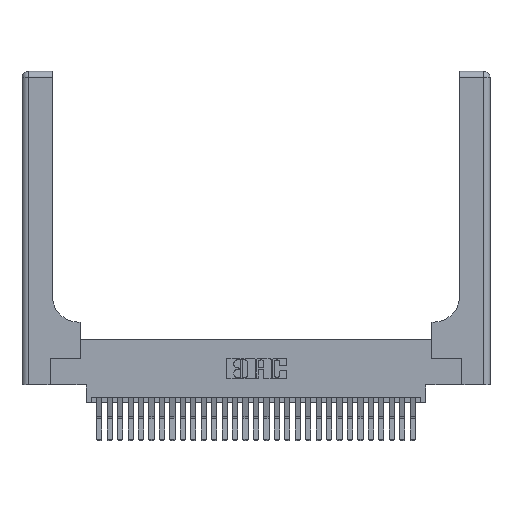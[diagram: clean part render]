
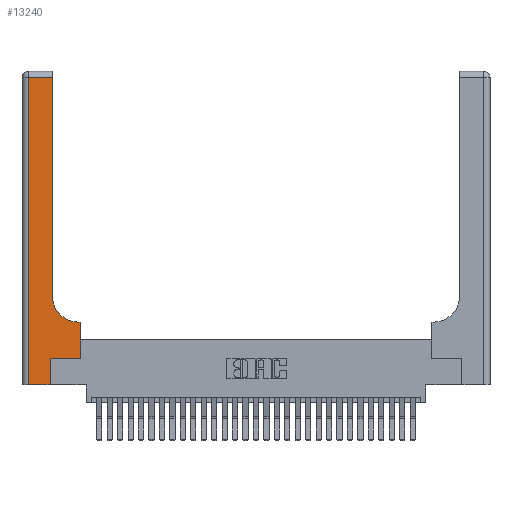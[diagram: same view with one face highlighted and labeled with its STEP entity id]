
A CAD part, top view. The second image highlights one B-rep face of the part: STEP entity #13240.
In plain terms, the highlighted planar face has unit normal (0, 0, 1).
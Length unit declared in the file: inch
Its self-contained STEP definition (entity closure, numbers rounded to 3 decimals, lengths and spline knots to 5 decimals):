
#451 = DIRECTION ( 'NONE',  ( 0., 1., 0. ) ) ;
#740 = VERTEX_POINT ( 'NONE', #11232 ) ;
#1038 = VERTEX_POINT ( 'NONE', #19438 ) ;
#1627 = CARTESIAN_POINT ( 'NONE',  ( 0.5585, 0.25, 0.37 ) ) ;
#1645 = CARTESIAN_POINT ( 'NONE',  ( 0.2915, 3., 0.37 ) ) ;
#1821 = ORIENTED_EDGE ( 'NONE', *, *, #20542, .T. ) ;
#2801 = VECTOR ( 'NONE', #21029, 39.37008 ) ;
#3345 = ORIENTED_EDGE ( 'NONE', *, *, #9586, .T. ) ;
#5707 = VERTEX_POINT ( 'NONE', #18124 ) ;
#5910 = CARTESIAN_POINT ( 'NONE',  ( 0., 3., 0.37 ) ) ;
#6053 = VERTEX_POINT ( 'NONE', #7316 ) ;
#6353 = ORIENTED_EDGE ( 'NONE', *, *, #28209, .T. ) ;
#6620 = EDGE_LOOP ( 'NONE', ( #1821, #24110, #27505, #6353, #18355, #17321, #18136, #19161, #3345 ) ) ;
#6633 = DIRECTION ( 'NONE',  ( 1., 0., 0. ) ) ;
#7102 = EDGE_CURVE ( 'NONE', #10843, #10697, #19552, .T. ) ;
#7316 = CARTESIAN_POINT ( 'NONE',  ( 0.269, 0., 0.37 ) ) ;
#7738 = EDGE_CURVE ( 'NONE', #5707, #740, #7755, .T. ) ;
#7755 = LINE ( 'NONE', #25929, #27038 ) ;
#8077 = VECTOR ( 'NONE', #451, 39.37008 ) ;
#8342 = DIRECTION ( 'NONE',  ( -1., 0., 0. ) ) ;
#9436 = DIRECTION ( 'NONE',  ( 0., -1., 0. ) ) ;
#9585 = VECTOR ( 'NONE', #30864, 39.37008 ) ;
#9586 = EDGE_CURVE ( 'NONE', #740, #12285, #17113, .T. ) ;
#9631 = EDGE_CURVE ( 'NONE', #1038, #24545, #27657, .T. ) ;
#10028 = LINE ( 'NONE', #1645, #2801 ) ;
#10697 = VERTEX_POINT ( 'NONE', #1627 ) ;
#10843 = VERTEX_POINT ( 'NONE', #31028 ) ;
#11232 = CARTESIAN_POINT ( 'NONE',  ( 0.5415, 0.6, 0.37 ) ) ;
#11270 = AXIS2_PLACEMENT_3D ( 'NONE', #28506, #14061, #30880 ) ;
#11654 = CARTESIAN_POINT ( 'NONE',  ( 0., 2.94, 0.37 ) ) ;
#12285 = VERTEX_POINT ( 'NONE', #24727 ) ;
#13110 = VECTOR ( 'NONE', #25637, 39.37008 ) ;
#13180 = FACE_OUTER_BOUND ( 'NONE', #6620, .T. ) ;
#13240 = ADVANCED_FACE ( 'NONE', ( #13180 ), #15536, .F. ) ;
#13889 = DIRECTION ( 'NONE',  ( -1., 0., 0. ) ) ;
#14061 = DIRECTION ( 'NONE',  ( 0., 0., -1. ) ) ;
#14318 = CARTESIAN_POINT ( 'NONE',  ( 0.06, 0., 0.37 ) ) ;
#14535 = LINE ( 'NONE', #29373, #8077 ) ;
#14829 = VECTOR ( 'NONE', #9436, 39.37008 ) ;
#15211 = LINE ( 'NONE', #11654, #9585 ) ;
#15536 = PLANE ( 'NONE',  #26261 ) ;
#17113 = CIRCLE ( 'NONE', #11270, 0.25 ) ;
#17321 = ORIENTED_EDGE ( 'NONE', *, *, #7102, .T. ) ;
#17659 = VERTEX_POINT ( 'NONE', #22381 ) ;
#18124 = CARTESIAN_POINT ( 'NONE',  ( 0.5585, 0.6, 0.37 ) ) ;
#18136 = ORIENTED_EDGE ( 'NONE', *, *, #20824, .T. ) ;
#18355 = ORIENTED_EDGE ( 'NONE', *, *, #22692, .T. ) ;
#18679 = CARTESIAN_POINT ( 'NONE',  ( 0., 0., 0.37 ) ) ;
#18980 = CARTESIAN_POINT ( 'NONE',  ( 0.269, 0., 0.37 ) ) ;
#19042 = CARTESIAN_POINT ( 'NONE',  ( 0.06, 3., 0.37 ) ) ;
#19161 = ORIENTED_EDGE ( 'NONE', *, *, #7738, .T. ) ;
#19438 = CARTESIAN_POINT ( 'NONE',  ( 0.06, 2.94, 0.37 ) ) ;
#19552 = LINE ( 'NONE', #20818, #13110 ) ;
#20542 = EDGE_CURVE ( 'NONE', #12285, #17659, #10028, .T. ) ;
#20818 = CARTESIAN_POINT ( 'NONE',  ( 0.269, 0.25, 0.37 ) ) ;
#20824 = EDGE_CURVE ( 'NONE', #10697, #5707, #14535, .T. ) ;
#21029 = DIRECTION ( 'NONE',  ( 0., 1., 0. ) ) ;
#21130 = VECTOR ( 'NONE', #6633, 39.37008 ) ;
#21779 = EDGE_CURVE ( 'NONE', #17659, #1038, #15211, .T. ) ;
#22381 = CARTESIAN_POINT ( 'NONE',  ( 0.2915, 2.94, 0.37 ) ) ;
#22692 = EDGE_CURVE ( 'NONE', #6053, #10843, #27998, .T. ) ;
#22846 = DIRECTION ( 'NONE',  ( 0., 0., -1. ) ) ;
#24110 = ORIENTED_EDGE ( 'NONE', *, *, #21779, .T. ) ;
#24545 = VERTEX_POINT ( 'NONE', #14318 ) ;
#24727 = CARTESIAN_POINT ( 'NONE',  ( 0.2915, 0.85, 0.37 ) ) ;
#25637 = DIRECTION ( 'NONE',  ( 1., 0., 0. ) ) ;
#25929 = CARTESIAN_POINT ( 'NONE',  ( 0.2915, 0.6, 0.37 ) ) ;
#26261 = AXIS2_PLACEMENT_3D ( 'NONE', #5910, #22846, #8342 ) ;
#27038 = VECTOR ( 'NONE', #13889, 39.37008 ) ;
#27247 = VECTOR ( 'NONE', #31025, 39.37008 ) ;
#27493 = LINE ( 'NONE', #18679, #21130 ) ;
#27505 = ORIENTED_EDGE ( 'NONE', *, *, #9631, .T. ) ;
#27657 = LINE ( 'NONE', #19042, #14829 ) ;
#27998 = LINE ( 'NONE', #18980, #27247 ) ;
#28209 = EDGE_CURVE ( 'NONE', #24545, #6053, #27493, .T. ) ;
#28506 = CARTESIAN_POINT ( 'NONE',  ( 0.5415, 0.85, 0.37 ) ) ;
#29373 = CARTESIAN_POINT ( 'NONE',  ( 0.5585, 0.25, 0.37 ) ) ;
#30864 = DIRECTION ( 'NONE',  ( -1., 0., 0. ) ) ;
#30880 = DIRECTION ( 'NONE',  ( 1., 0., 0. ) ) ;
#31025 = DIRECTION ( 'NONE',  ( 0., 1., 0. ) ) ;
#31028 = CARTESIAN_POINT ( 'NONE',  ( 0.269, 0.25, 0.37 ) ) ;
